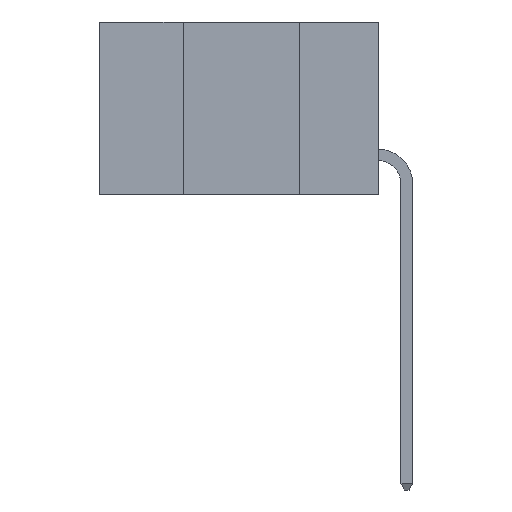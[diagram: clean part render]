
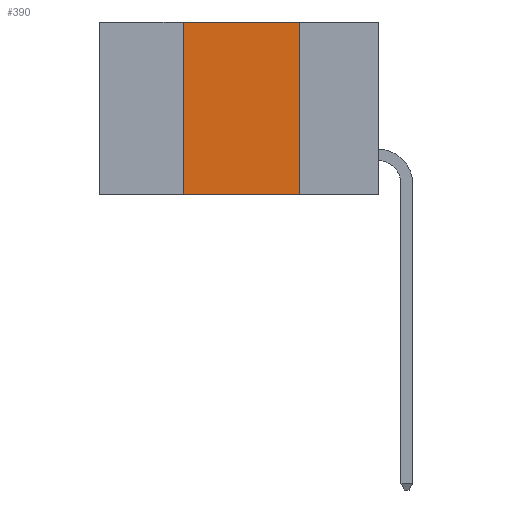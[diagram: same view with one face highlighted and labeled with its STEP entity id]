
A CAD part, left-side view. The second image highlights one B-rep face of the part: STEP entity #390.
In plain terms, the highlighted planar face has unit normal (-1, 0, 0).
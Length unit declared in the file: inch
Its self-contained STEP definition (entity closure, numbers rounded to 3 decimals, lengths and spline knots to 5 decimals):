
#16 = ORIENTED_EDGE ( 'NONE', *, *, #1996, .T. ) ;
#62 = DIRECTION ( 'NONE',  ( 0., 0., 1. ) ) ;
#269 = VECTOR ( 'NONE', #5231, 39.37008 ) ;
#390 = ADVANCED_FACE ( 'NONE', ( #432 ), #1051, .F. ) ;
#432 = FACE_OUTER_BOUND ( 'NONE', #927, .T. ) ;
#541 = EDGE_CURVE ( 'NONE', #3994, #8312, #1227, .T. ) ;
#848 = EDGE_CURVE ( 'NONE', #4003, #3994, #6112, .T. ) ;
#891 = VERTEX_POINT ( 'NONE', #5307 ) ;
#927 = EDGE_LOOP ( 'NONE', ( #6136, #5087, #1954, #16 ) ) ;
#1051 = PLANE ( 'NONE',  #6828 ) ;
#1227 = LINE ( 'NONE', #2671, #6409 ) ;
#1465 = CARTESIAN_POINT ( 'NONE',  ( 0., 0.6, 0. ) ) ;
#1954 = ORIENTED_EDGE ( 'NONE', *, *, #848, .F. ) ;
#1996 = EDGE_CURVE ( 'NONE', #4003, #891, #7226, .T. ) ;
#2022 = DIRECTION ( 'NONE',  ( 0., -1., 0. ) ) ;
#2134 = DIRECTION ( 'NONE',  ( 1., 0., 0. ) ) ;
#2530 = VECTOR ( 'NONE', #62, 39.37008 ) ;
#2671 = CARTESIAN_POINT ( 'NONE',  ( 0., 0.6, 0. ) ) ;
#2890 = CARTESIAN_POINT ( 'NONE',  ( 0., 0.42, -0.37 ) ) ;
#3318 = LINE ( 'NONE', #7654, #6558 ) ;
#3620 = DIRECTION ( 'NONE',  ( 0., 0., -1. ) ) ;
#3994 = VERTEX_POINT ( 'NONE', #7152 ) ;
#4003 = VERTEX_POINT ( 'NONE', #2890 ) ;
#4362 = CARTESIAN_POINT ( 'NONE',  ( 0., 0.17, 0. ) ) ;
#5087 = ORIENTED_EDGE ( 'NONE', *, *, #541, .F. ) ;
#5231 = DIRECTION ( 'NONE',  ( 0., -1., 0. ) ) ;
#5307 = CARTESIAN_POINT ( 'NONE',  ( 0., 0.17, -0.37 ) ) ;
#6076 = CARTESIAN_POINT ( 'NONE',  ( 0., 0.42, -0.37 ) ) ;
#6112 = LINE ( 'NONE', #6076, #2530 ) ;
#6136 = ORIENTED_EDGE ( 'NONE', *, *, #7685, .F. ) ;
#6250 = CARTESIAN_POINT ( 'NONE',  ( 0., 0.6, -0.37 ) ) ;
#6409 = VECTOR ( 'NONE', #2022, 39.37008 ) ;
#6558 = VECTOR ( 'NONE', #7661, 39.37008 ) ;
#6828 = AXIS2_PLACEMENT_3D ( 'NONE', #1465, #2134, #3620 ) ;
#7152 = CARTESIAN_POINT ( 'NONE',  ( 0., 0.42, 0. ) ) ;
#7226 = LINE ( 'NONE', #6250, #269 ) ;
#7654 = CARTESIAN_POINT ( 'NONE',  ( 0., 0.17, -0.37 ) ) ;
#7661 = DIRECTION ( 'NONE',  ( 0., 0., -1. ) ) ;
#7685 = EDGE_CURVE ( 'NONE', #8312, #891, #3318, .T. ) ;
#8312 = VERTEX_POINT ( 'NONE', #4362 ) ;
